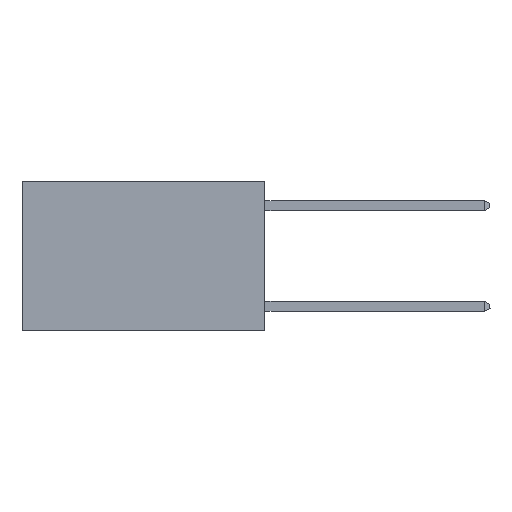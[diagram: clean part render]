
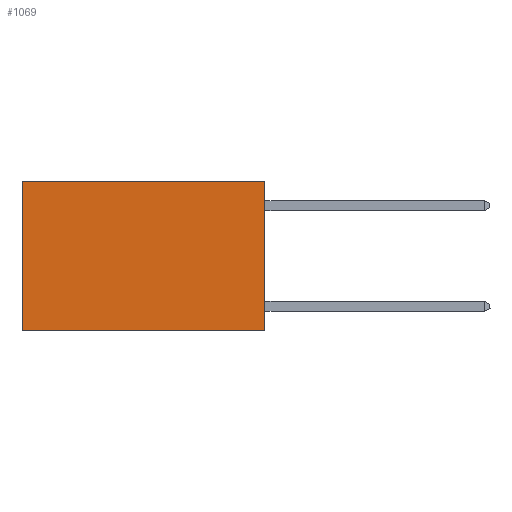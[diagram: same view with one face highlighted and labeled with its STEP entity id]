
A CAD part, left-side view. The second image highlights one B-rep face of the part: STEP entity #1069.
In plain terms, the highlighted planar face has unit normal (-1, 0, 0).
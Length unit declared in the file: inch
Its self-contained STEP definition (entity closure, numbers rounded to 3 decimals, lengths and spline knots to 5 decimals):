
#68 = VECTOR ( 'NONE', #519, 39.37008 ) ;
#519 = DIRECTION ( 'NONE',  ( 0., 1., 0. ) ) ;
#887 = EDGE_CURVE ( 'NONE', #7996, #3014, #2996, .T. ) ;
#941 = CARTESIAN_POINT ( 'NONE',  ( 0.2625, 0., 0. ) ) ;
#1069 = ADVANCED_FACE ( 'NONE', ( #7338 ), #9963, .F. ) ;
#1673 = DIRECTION ( 'NONE',  ( 0., 0., -1. ) ) ;
#1807 = LINE ( 'NONE', #6779, #6456 ) ;
#2080 = VECTOR ( 'NONE', #9849, 39.37008 ) ;
#2298 = EDGE_LOOP ( 'NONE', ( #3912, #6130, #12312, #5691 ) ) ;
#2314 = EDGE_CURVE ( 'NONE', #3014, #11390, #11162, .T. ) ;
#2996 = LINE ( 'NONE', #941, #68 ) ;
#3014 = VERTEX_POINT ( 'NONE', #5802 ) ;
#3597 = CARTESIAN_POINT ( 'NONE',  ( 0.2625, 0., 0. ) ) ;
#3912 = ORIENTED_EDGE ( 'NONE', *, *, #2314, .T. ) ;
#3964 = AXIS2_PLACEMENT_3D ( 'NONE', #10044, #9801, #9790 ) ;
#5155 = EDGE_CURVE ( 'NONE', #8705, #11390, #1807, .T. ) ;
#5691 = ORIENTED_EDGE ( 'NONE', *, *, #887, .T. ) ;
#5802 = CARTESIAN_POINT ( 'NONE',  ( 0.2625, 0.6, 0. ) ) ;
#6111 = VECTOR ( 'NONE', #1673, 39.37008 ) ;
#6130 = ORIENTED_EDGE ( 'NONE', *, *, #5155, .F. ) ;
#6456 = VECTOR ( 'NONE', #9632, 39.37008 ) ;
#6779 = CARTESIAN_POINT ( 'NONE',  ( 0.2625, 0., -0.37 ) ) ;
#7338 = FACE_OUTER_BOUND ( 'NONE', #2298, .T. ) ;
#7536 = EDGE_CURVE ( 'NONE', #7996, #8705, #9843, .T. ) ;
#7996 = VERTEX_POINT ( 'NONE', #3597 ) ;
#8186 = CARTESIAN_POINT ( 'NONE',  ( 0.2625, 0., -0.37 ) ) ;
#8705 = VERTEX_POINT ( 'NONE', #8186 ) ;
#8998 = CARTESIAN_POINT ( 'NONE',  ( 0.2625, 0.6, -0.37 ) ) ;
#9632 = DIRECTION ( 'NONE',  ( 0., 1., 0. ) ) ;
#9790 = DIRECTION ( 'NONE',  ( 0., 0., -1. ) ) ;
#9801 = DIRECTION ( 'NONE',  ( 1., 0., 0. ) ) ;
#9843 = LINE ( 'NONE', #10784, #2080 ) ;
#9849 = DIRECTION ( 'NONE',  ( 0., 0., -1. ) ) ;
#9963 = PLANE ( 'NONE',  #3964 ) ;
#10044 = CARTESIAN_POINT ( 'NONE',  ( 0.2625, 0., 0. ) ) ;
#10784 = CARTESIAN_POINT ( 'NONE',  ( 0.2625, 0., 0. ) ) ;
#11162 = LINE ( 'NONE', #12296, #6111 ) ;
#11390 = VERTEX_POINT ( 'NONE', #8998 ) ;
#12296 = CARTESIAN_POINT ( 'NONE',  ( 0.2625, 0.6, 0. ) ) ;
#12312 = ORIENTED_EDGE ( 'NONE', *, *, #7536, .F. ) ;
